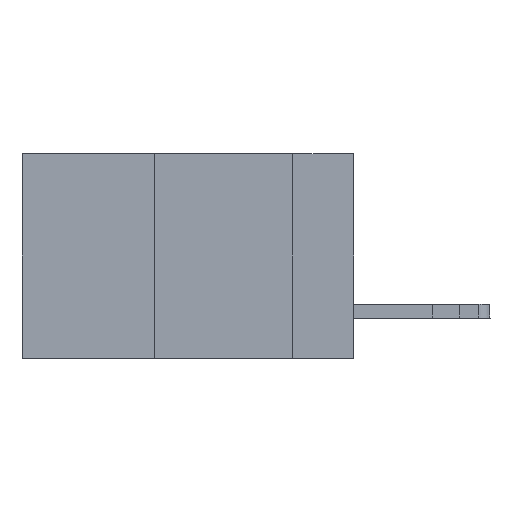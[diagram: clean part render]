
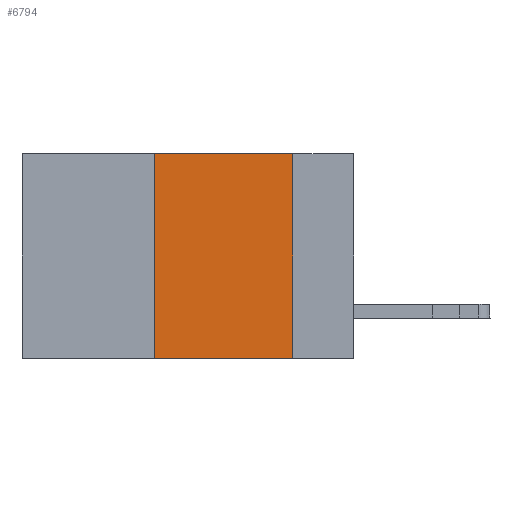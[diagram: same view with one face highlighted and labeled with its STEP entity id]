
A CAD part, left-side view. The second image highlights one B-rep face of the part: STEP entity #6794.
In plain terms, the highlighted planar face has unit normal (-1, 0, 0).
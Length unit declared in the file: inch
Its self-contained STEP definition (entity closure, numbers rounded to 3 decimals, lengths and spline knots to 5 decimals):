
#1092 = EDGE_CURVE ( 'NONE', #20187, #6515, #27007, .T. ) ;
#3108 = DIRECTION ( 'NONE',  ( 0., 0., -1. ) ) ;
#3868 = VERTEX_POINT ( 'NONE', #13558 ) ;
#4828 = LINE ( 'NONE', #30715, #24274 ) ;
#5317 = ORIENTED_EDGE ( 'NONE', *, *, #24904, .F. ) ;
#6403 = CARTESIAN_POINT ( 'NONE',  ( 0., 0.36, 0. ) ) ;
#6515 = VERTEX_POINT ( 'NONE', #11937 ) ;
#6794 = ADVANCED_FACE ( 'NONE', ( #15657 ), #13025, .F. ) ;
#7558 = VECTOR ( 'NONE', #11978, 39.37008 ) ;
#11937 = CARTESIAN_POINT ( 'NONE',  ( 0., 0.11, -0.37 ) ) ;
#11978 = DIRECTION ( 'NONE',  ( 0., -1., 0. ) ) ;
#12000 = ORIENTED_EDGE ( 'NONE', *, *, #13573, .F. ) ;
#13010 = CARTESIAN_POINT ( 'NONE',  ( 0., 0.36, -0.37 ) ) ;
#13025 = PLANE ( 'NONE',  #20091 ) ;
#13558 = CARTESIAN_POINT ( 'NONE',  ( 0., 0.11, 0. ) ) ;
#13573 = EDGE_CURVE ( 'NONE', #20187, #32250, #26766, .T. ) ;
#14563 = DIRECTION ( 'NONE',  ( 0., 0., 1. ) ) ;
#15657 = FACE_OUTER_BOUND ( 'NONE', #30853, .T. ) ;
#16946 = CARTESIAN_POINT ( 'NONE',  ( 0., 0.6, -0.37 ) ) ;
#17085 = CARTESIAN_POINT ( 'NONE',  ( 0., 0.6, 0. ) ) ;
#17907 = ORIENTED_EDGE ( 'NONE', *, *, #26557, .F. ) ;
#18015 = DIRECTION ( 'NONE',  ( 0., 0., -1. ) ) ;
#18199 = DIRECTION ( 'NONE',  ( 1., 0., 0. ) ) ;
#19642 = DIRECTION ( 'NONE',  ( 0., -1., 0. ) ) ;
#19935 = VECTOR ( 'NONE', #14563, 39.37008 ) ;
#20091 = AXIS2_PLACEMENT_3D ( 'NONE', #30903, #18199, #3108 ) ;
#20187 = VERTEX_POINT ( 'NONE', #13010 ) ;
#22131 = CARTESIAN_POINT ( 'NONE',  ( 0., 0.36, 0. ) ) ;
#24274 = VECTOR ( 'NONE', #18015, 39.37008 ) ;
#24904 = EDGE_CURVE ( 'NONE', #32250, #3868, #29514, .T. ) ;
#26557 = EDGE_CURVE ( 'NONE', #3868, #6515, #4828, .T. ) ;
#26766 = LINE ( 'NONE', #22131, #19935 ) ;
#27007 = LINE ( 'NONE', #16946, #7558 ) ;
#28708 = VECTOR ( 'NONE', #19642, 39.37008 ) ;
#29514 = LINE ( 'NONE', #17085, #28708 ) ;
#30715 = CARTESIAN_POINT ( 'NONE',  ( 0., 0.11, 0. ) ) ;
#30853 = EDGE_LOOP ( 'NONE', ( #17907, #5317, #12000, #32257 ) ) ;
#30903 = CARTESIAN_POINT ( 'NONE',  ( 0., 0.6, 0. ) ) ;
#32250 = VERTEX_POINT ( 'NONE', #6403 ) ;
#32257 = ORIENTED_EDGE ( 'NONE', *, *, #1092, .T. ) ;
